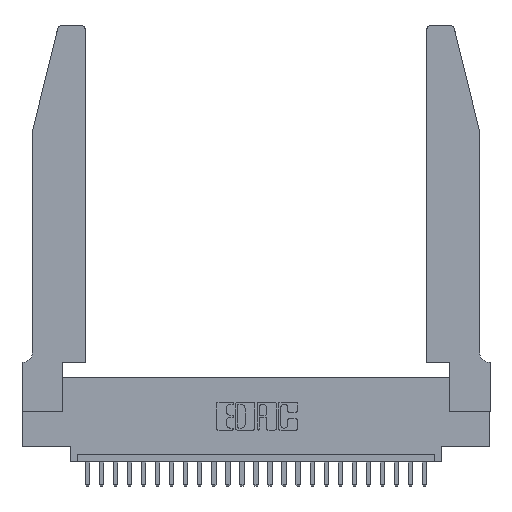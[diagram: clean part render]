
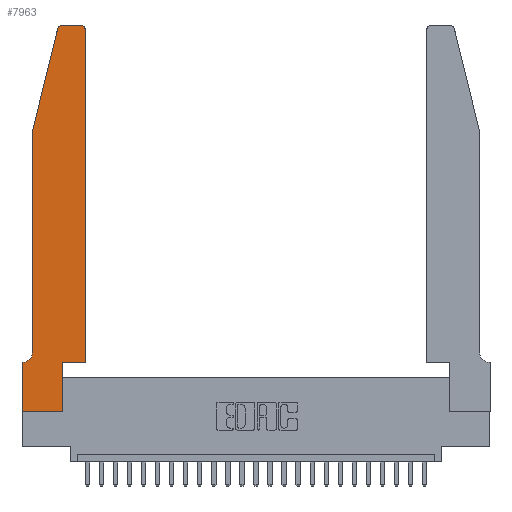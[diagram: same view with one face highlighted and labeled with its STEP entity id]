
A CAD part, top view. The second image highlights one B-rep face of the part: STEP entity #7963.
In plain terms, the highlighted planar face has unit normal (0, 0, 1).
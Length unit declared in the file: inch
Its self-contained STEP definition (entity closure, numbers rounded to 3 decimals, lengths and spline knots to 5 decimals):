
#71 = CARTESIAN_POINT ( 'NONE',  ( 0.25487, 2.72718, 0.37 ) ) ;
#137 = CARTESIAN_POINT ( 'NONE',  ( 0.4505, 0.35, 0.37 ) ) ;
#290 = LINE ( 'NONE', #20991, #4414 ) ;
#615 = CARTESIAN_POINT ( 'NONE',  ( 0.4205, 2.72, 0.37 ) ) ;
#707 = AXIS2_PLACEMENT_3D ( 'NONE', #5491, #15737, #21626 ) ;
#863 = CARTESIAN_POINT ( 'NONE',  ( 0., 0., 0.37 ) ) ;
#971 = ORIENTED_EDGE ( 'NONE', *, *, #11775, .T. ) ;
#1165 = VERTEX_POINT ( 'NONE', #18178 ) ;
#1286 = CARTESIAN_POINT ( 'NONE',  ( 0.2865, 0., 0.37 ) ) ;
#1589 = PLANE ( 'NONE',  #707 ) ;
#1846 = EDGE_CURVE ( 'NONE', #16014, #22406, #17176, .T. ) ;
#1860 = CARTESIAN_POINT ( 'NONE',  ( 0.0055, 0.42, 0.37 ) ) ;
#1941 = DIRECTION ( 'NONE',  ( -1., 0., 0. ) ) ;
#2401 = VERTEX_POINT ( 'NONE', #6518 ) ;
#2666 = ORIENTED_EDGE ( 'NONE', *, *, #7627, .T. ) ;
#2784 = CARTESIAN_POINT ( 'NONE',  ( 0.4505, 0.35, 0.37 ) ) ;
#2918 = DIRECTION ( 'NONE',  ( 0., 0., 1. ) ) ;
#3005 = VECTOR ( 'NONE', #7316, 39.37008 ) ;
#3192 = ORIENTED_EDGE ( 'NONE', *, *, #10578, .T. ) ;
#3384 = ORIENTED_EDGE ( 'NONE', *, *, #1846, .T. ) ;
#3457 = VERTEX_POINT ( 'NONE', #71 ) ;
#3459 = VECTOR ( 'NONE', #18137, 39.37008 ) ;
#3776 = CARTESIAN_POINT ( 'NONE',  ( 0.0755, 2., 0.37 ) ) ;
#3892 = DIRECTION ( 'NONE',  ( 0., 0., -1. ) ) ;
#4162 = ORIENTED_EDGE ( 'NONE', *, *, #19743, .T. ) ;
#4414 = VECTOR ( 'NONE', #24996, 39.37008 ) ;
#5090 = ORIENTED_EDGE ( 'NONE', *, *, #10962, .T. ) ;
#5296 = VERTEX_POINT ( 'NONE', #137 ) ;
#5491 = CARTESIAN_POINT ( 'NONE',  ( 0., 0.35, 0.37 ) ) ;
#5661 = VERTEX_POINT ( 'NONE', #9113 ) ;
#5745 = CARTESIAN_POINT ( 'NONE',  ( 0.284, 2.72, 0.37 ) ) ;
#5887 = ORIENTED_EDGE ( 'NONE', *, *, #26058, .T. ) ;
#5947 = LINE ( 'NONE', #17126, #21409 ) ;
#6376 = CARTESIAN_POINT ( 'NONE',  ( 0., 0.35, 0.37 ) ) ;
#6518 = CARTESIAN_POINT ( 'NONE',  ( 0.284, 2.75, 0.37 ) ) ;
#6707 = CARTESIAN_POINT ( 'NONE',  ( 0.0755, 0.42, 0.37 ) ) ;
#6800 = VERTEX_POINT ( 'NONE', #6376 ) ;
#7037 = CIRCLE ( 'NONE', #11369, 0.03 ) ;
#7316 = DIRECTION ( 'NONE',  ( 0., 1., 0. ) ) ;
#7605 = AXIS2_PLACEMENT_3D ( 'NONE', #1860, #3892, #1941 ) ;
#7627 = EDGE_CURVE ( 'NONE', #2401, #3457, #18189, .T. ) ;
#7963 = ADVANCED_FACE ( 'NONE', ( #25205 ), #1589, .T. ) ;
#9113 = CARTESIAN_POINT ( 'NONE',  ( 0.4205, 2.75, 0.37 ) ) ;
#10578 = EDGE_CURVE ( 'NONE', #5296, #17340, #17531, .T. ) ;
#10919 = CARTESIAN_POINT ( 'NONE',  ( 0.0755, 2., 0.37 ) ) ;
#10962 = EDGE_CURVE ( 'NONE', #19904, #5296, #13732, .T. ) ;
#11369 = AXIS2_PLACEMENT_3D ( 'NONE', #615, #2918, #19074 ) ;
#11511 = EDGE_CURVE ( 'NONE', #17698, #1165, #19996, .T. ) ;
#11775 = EDGE_CURVE ( 'NONE', #3457, #20266, #19972, .T. ) ;
#12798 = ORIENTED_EDGE ( 'NONE', *, *, #11511, .T. ) ;
#13352 = DIRECTION ( 'NONE',  ( -1., 0., 0. ) ) ;
#13728 = DIRECTION ( 'NONE',  ( 0., 0., 1. ) ) ;
#13732 = LINE ( 'NONE', #2784, #16858 ) ;
#14074 = EDGE_LOOP ( 'NONE', ( #24524, #2666, #971, #4162, #12798, #5887, #14952, #3384, #18489, #5090, #3192, #19605 ) ) ;
#14344 = VECTOR ( 'NONE', #21320, 39.37008 ) ;
#14952 = ORIENTED_EDGE ( 'NONE', *, *, #16562, .T. ) ;
#15538 = DIRECTION ( 'NONE',  ( -1., 0., 0. ) ) ;
#15737 = DIRECTION ( 'NONE',  ( 0., 0., 1. ) ) ;
#16014 = VERTEX_POINT ( 'NONE', #19309 ) ;
#16255 = VECTOR ( 'NONE', #17046, 39.37008 ) ;
#16562 = EDGE_CURVE ( 'NONE', #6800, #16014, #23785, .T. ) ;
#16705 = DIRECTION ( 'NONE',  ( -0.239, -0.971, 0. ) ) ;
#16858 = VECTOR ( 'NONE', #16916, 39.37008 ) ;
#16916 = DIRECTION ( 'NONE',  ( 1., 0., 0. ) ) ;
#17046 = DIRECTION ( 'NONE',  ( 1., 0., 0. ) ) ;
#17126 = CARTESIAN_POINT ( 'NONE',  ( 0.0755, 0.35, 0.37 ) ) ;
#17140 = VECTOR ( 'NONE', #16705, 39.37008 ) ;
#17176 = LINE ( 'NONE', #863, #16255 ) ;
#17340 = VERTEX_POINT ( 'NONE', #18552 ) ;
#17531 = LINE ( 'NONE', #19699, #3005 ) ;
#17698 = VERTEX_POINT ( 'NONE', #6707 ) ;
#18137 = DIRECTION ( 'NONE',  ( 0., -1., 0. ) ) ;
#18178 = CARTESIAN_POINT ( 'NONE',  ( 0.0055, 0.35, 0.37 ) ) ;
#18189 = CIRCLE ( 'NONE', #20683, 0.03 ) ;
#18489 = ORIENTED_EDGE ( 'NONE', *, *, #24741, .T. ) ;
#18552 = CARTESIAN_POINT ( 'NONE',  ( 0.4505, 2.72, 0.37 ) ) ;
#18933 = EDGE_CURVE ( 'NONE', #5661, #2401, #19607, .T. ) ;
#19074 = DIRECTION ( 'NONE',  ( 1., 0., 0. ) ) ;
#19309 = CARTESIAN_POINT ( 'NONE',  ( 0., 0., 0.37 ) ) ;
#19365 = CARTESIAN_POINT ( 'NONE',  ( 0., 0., 0.37 ) ) ;
#19605 = ORIENTED_EDGE ( 'NONE', *, *, #24066, .T. ) ;
#19607 = LINE ( 'NONE', #24913, #21172 ) ;
#19609 = DIRECTION ( 'NONE',  ( 1., 0., 0. ) ) ;
#19699 = CARTESIAN_POINT ( 'NONE',  ( 0.4505, 0.35, 0.37 ) ) ;
#19743 = EDGE_CURVE ( 'NONE', #20266, #17698, #25194, .T. ) ;
#19904 = VERTEX_POINT ( 'NONE', #20859 ) ;
#19972 = LINE ( 'NONE', #10919, #17140 ) ;
#19996 = CIRCLE ( 'NONE', #7605, 0.07 ) ;
#20266 = VERTEX_POINT ( 'NONE', #24673 ) ;
#20683 = AXIS2_PLACEMENT_3D ( 'NONE', #5745, #13728, #19609 ) ;
#20859 = CARTESIAN_POINT ( 'NONE',  ( 0.2865, 0.35, 0.37 ) ) ;
#20991 = CARTESIAN_POINT ( 'NONE',  ( 0.2865, 0.35, 0.37 ) ) ;
#21172 = VECTOR ( 'NONE', #15538, 39.37008 ) ;
#21320 = DIRECTION ( 'NONE',  ( 0., -1., 0. ) ) ;
#21409 = VECTOR ( 'NONE', #13352, 39.37008 ) ;
#21626 = DIRECTION ( 'NONE',  ( 1., 0., 0. ) ) ;
#22406 = VERTEX_POINT ( 'NONE', #1286 ) ;
#23785 = LINE ( 'NONE', #19365, #14344 ) ;
#24066 = EDGE_CURVE ( 'NONE', #17340, #5661, #7037, .T. ) ;
#24524 = ORIENTED_EDGE ( 'NONE', *, *, #18933, .T. ) ;
#24673 = CARTESIAN_POINT ( 'NONE',  ( 0.0755, 2., 0.37 ) ) ;
#24741 = EDGE_CURVE ( 'NONE', #22406, #19904, #290, .T. ) ;
#24913 = CARTESIAN_POINT ( 'NONE',  ( 0.2605, 2.75, 0.37 ) ) ;
#24996 = DIRECTION ( 'NONE',  ( 0., 1., 0. ) ) ;
#25194 = LINE ( 'NONE', #3776, #3459 ) ;
#25205 = FACE_OUTER_BOUND ( 'NONE', #14074, .T. ) ;
#26058 = EDGE_CURVE ( 'NONE', #1165, #6800, #5947, .T. ) ;
